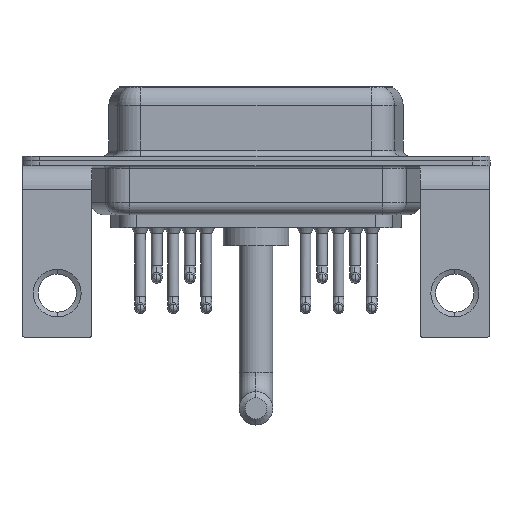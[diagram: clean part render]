
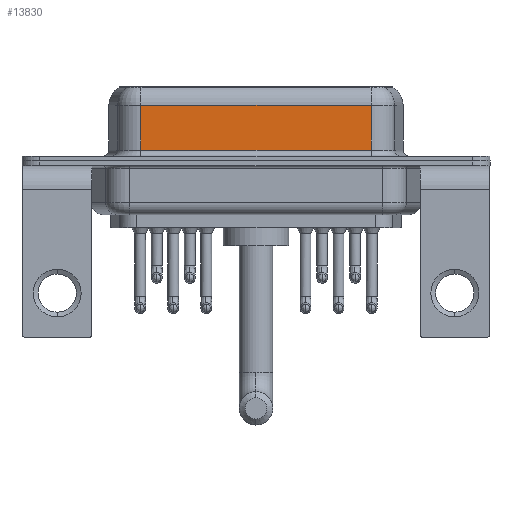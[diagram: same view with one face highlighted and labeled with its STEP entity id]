
A CAD part, front view. The second image highlights one B-rep face of the part: STEP entity #13830.
In plain terms, the highlighted planar face has unit normal (0, -1, 0).
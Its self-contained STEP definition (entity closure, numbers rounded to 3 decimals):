
#197 = CARTESIAN_POINT ( 'NONE',  ( 26.287, -3.95, 4.65 ) ) ;
#569 = EDGE_CURVE ( 'NONE', #3555, #14478, #10750, .T. ) ;
#1020 = VERTEX_POINT ( 'NONE', #197 ) ;
#2219 = CARTESIAN_POINT ( 'NONE',  ( 26.287, -3.95, 6.4 ) ) ;
#3025 = EDGE_LOOP ( 'NONE', ( #11335, #18973, #6700, #11237 ) ) ;
#3526 = CARTESIAN_POINT ( 'NONE',  ( 7.013, -3.95, 4.65 ) ) ;
#3555 = VERTEX_POINT ( 'NONE', #16833 ) ;
#3627 = EDGE_CURVE ( 'NONE', #1020, #14478, #14174, .T. ) ;
#4769 = DIRECTION ( 'NONE',  ( 1., 0., 0. ) ) ;
#5468 = VECTOR ( 'NONE', #4769, 1000. ) ;
#5575 = DIRECTION ( 'NONE',  ( -1., 0., 0. ) ) ;
#6700 = ORIENTED_EDGE ( 'NONE', *, *, #19328, .T. ) ;
#6754 = DIRECTION ( 'NONE',  ( 0., 1., 0. ) ) ;
#7167 = EDGE_CURVE ( 'NONE', #1020, #10542, #18109, .T. ) ;
#7729 = CARTESIAN_POINT ( 'NONE',  ( 26.287, -3.95, 0.9 ) ) ;
#7972 = DIRECTION ( 'NONE',  ( 0., 0., -1. ) ) ;
#8096 = DIRECTION ( 'NONE',  ( 0., 0., -1. ) ) ;
#10542 = VERTEX_POINT ( 'NONE', #3526 ) ;
#10596 = PLANE ( 'NONE',  #19375 ) ;
#10750 = LINE ( 'NONE', #7729, #5468 ) ;
#11158 = DIRECTION ( 'NONE',  ( 0., 0., 1. ) ) ;
#11237 = ORIENTED_EDGE ( 'NONE', *, *, #569, .T. ) ;
#11335 = ORIENTED_EDGE ( 'NONE', *, *, #3627, .F. ) ;
#11681 = CARTESIAN_POINT ( 'NONE',  ( 26.287, -3.95, 6.4 ) ) ;
#13477 = CARTESIAN_POINT ( 'NONE',  ( 26.287, -3.95, 4.65 ) ) ;
#13830 = ADVANCED_FACE ( 'NONE', ( #15670 ), #10596, .F. ) ;
#14174 = LINE ( 'NONE', #11681, #16888 ) ;
#14288 = VECTOR ( 'NONE', #5575, 1000. ) ;
#14478 = VERTEX_POINT ( 'NONE', #17697 ) ;
#15421 = CARTESIAN_POINT ( 'NONE',  ( 7.013, -3.95, 6.4 ) ) ;
#15670 = FACE_OUTER_BOUND ( 'NONE', #3025, .T. ) ;
#16000 = VECTOR ( 'NONE', #7972, 1000. ) ;
#16833 = CARTESIAN_POINT ( 'NONE',  ( 7.013, -3.95, 0.9 ) ) ;
#16888 = VECTOR ( 'NONE', #8096, 1000. ) ;
#16893 = LINE ( 'NONE', #15421, #16000 ) ;
#17697 = CARTESIAN_POINT ( 'NONE',  ( 26.287, -3.95, 0.9 ) ) ;
#18109 = LINE ( 'NONE', #13477, #14288 ) ;
#18973 = ORIENTED_EDGE ( 'NONE', *, *, #7167, .T. ) ;
#19328 = EDGE_CURVE ( 'NONE', #10542, #3555, #16893, .T. ) ;
#19375 = AXIS2_PLACEMENT_3D ( 'NONE', #2219, #6754, #11158 ) ;
